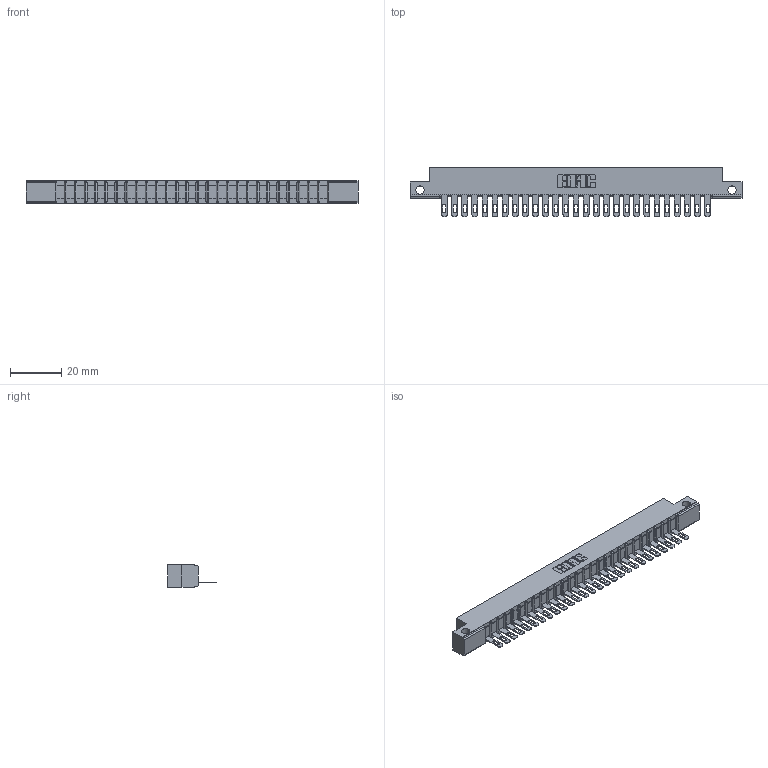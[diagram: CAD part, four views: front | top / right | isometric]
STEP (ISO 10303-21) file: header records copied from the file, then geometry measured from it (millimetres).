
FILE_DESCRIPTION (( 'STEP AP203' ), '1' );
FILE_NAME ('307-027-505-112.STEP', '2019-09-03T22:05:40', ( '' ), ( '' ), 'SwSTEP 2.0', 'SolidWorks 2016', '' );
FILE_SCHEMA (( 'CONFIG_CONTROL_DESIGN' ));
Length unit declared in the file: inch
Products named in the file (3): 307-027-505-112; 307-290-001_505; 307 Part_.128 Dia Side Mounting Holes
Assembly tree (28 placements, depth 2):
  307-027-505-112
    307 Part_.128 Dia Side Mounting Holes
    307-290-001_505  x27
Bounding box: 130 x 19.18 x 8.71 mm (x, y, z)
Volume: 8155.8 mm3; surface area: 12900.3 mm2
Topology: 28 solids, 28 shells, 1658 faces, 4697 edges, 3018 vertices
Faces by surface type: plane 1042, cylinder 560, sphere 56
Entity records: 24972 total; most frequent: CARTESIAN_POINT 4200, ORIENTED_EDGE 4186, DIRECTION 4095, EDGE_CURVE 2093, LINE 1597, VECTOR 1597, VERTEX_POINT 1354, AXIS2_PLACEMENT_3D 1249
